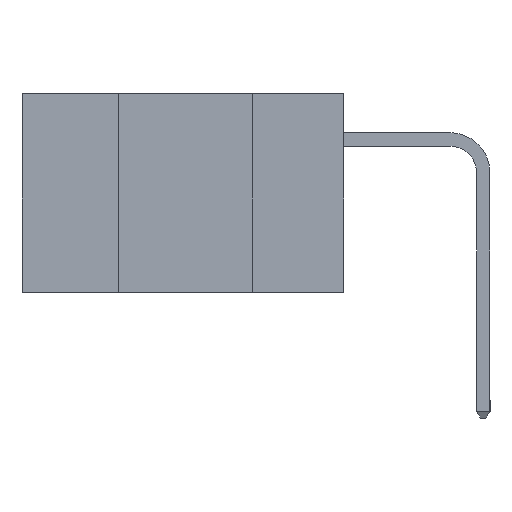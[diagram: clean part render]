
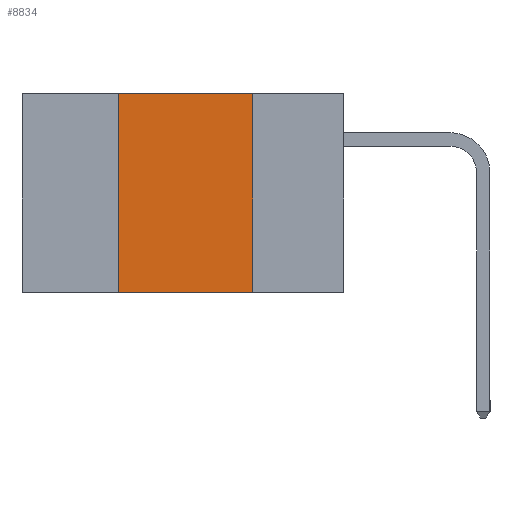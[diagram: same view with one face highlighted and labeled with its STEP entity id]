
A CAD part, left-side view. The second image highlights one B-rep face of the part: STEP entity #8834.
In plain terms, the highlighted planar face has unit normal (-1, 0, 0).
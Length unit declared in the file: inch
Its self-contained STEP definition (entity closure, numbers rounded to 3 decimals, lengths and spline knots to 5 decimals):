
#902 = DIRECTION ( 'NONE',  ( 0., 0., 1. ) ) ;
#1049 = VERTEX_POINT ( 'NONE', #13459 ) ;
#1389 = VECTOR ( 'NONE', #14288, 39.37008 ) ;
#2079 = CARTESIAN_POINT ( 'NONE',  ( 0., 0.42, -0.37 ) ) ;
#2468 = DIRECTION ( 'NONE',  ( 0., -1., 0. ) ) ;
#2486 = LINE ( 'NONE', #14290, #10947 ) ;
#2557 = CARTESIAN_POINT ( 'NONE',  ( 0., 0.17, -0.37 ) ) ;
#2605 = DIRECTION ( 'NONE',  ( 0., 0., -1. ) ) ;
#3822 = ORIENTED_EDGE ( 'NONE', *, *, #6301, .F. ) ;
#4528 = LINE ( 'NONE', #2079, #10556 ) ;
#4653 = ORIENTED_EDGE ( 'NONE', *, *, #6824, .T. ) ;
#5407 = VERTEX_POINT ( 'NONE', #14239 ) ;
#5997 = CARTESIAN_POINT ( 'NONE',  ( 0., 0.6, -0.37 ) ) ;
#6136 = AXIS2_PLACEMENT_3D ( 'NONE', #12160, #14434, #7365 ) ;
#6301 = EDGE_CURVE ( 'NONE', #1049, #13690, #12116, .T. ) ;
#6824 = EDGE_CURVE ( 'NONE', #5407, #13690, #13311, .T. ) ;
#6946 = FACE_OUTER_BOUND ( 'NONE', #10215, .T. ) ;
#7365 = DIRECTION ( 'NONE',  ( 0., 0., -1. ) ) ;
#8161 = VECTOR ( 'NONE', #2605, 39.37008 ) ;
#8766 = EDGE_CURVE ( 'NONE', #14682, #1049, #2486, .T. ) ;
#8834 = ADVANCED_FACE ( 'NONE', ( #6946 ), #13277, .F. ) ;
#10131 = CARTESIAN_POINT ( 'NONE',  ( 0., 0.42, 0. ) ) ;
#10215 = EDGE_LOOP ( 'NONE', ( #3822, #12230, #13303, #4653 ) ) ;
#10556 = VECTOR ( 'NONE', #902, 39.37008 ) ;
#10947 = VECTOR ( 'NONE', #2468, 39.37008 ) ;
#12116 = LINE ( 'NONE', #2557, #8161 ) ;
#12160 = CARTESIAN_POINT ( 'NONE',  ( 0., 0.6, 0. ) ) ;
#12230 = ORIENTED_EDGE ( 'NONE', *, *, #8766, .F. ) ;
#13277 = PLANE ( 'NONE',  #6136 ) ;
#13303 = ORIENTED_EDGE ( 'NONE', *, *, #14253, .F. ) ;
#13311 = LINE ( 'NONE', #5997, #1389 ) ;
#13459 = CARTESIAN_POINT ( 'NONE',  ( 0., 0.17, 0. ) ) ;
#13690 = VERTEX_POINT ( 'NONE', #14967 ) ;
#14239 = CARTESIAN_POINT ( 'NONE',  ( 0., 0.42, -0.37 ) ) ;
#14253 = EDGE_CURVE ( 'NONE', #5407, #14682, #4528, .T. ) ;
#14288 = DIRECTION ( 'NONE',  ( 0., -1., 0. ) ) ;
#14290 = CARTESIAN_POINT ( 'NONE',  ( 0., 0.6, 0. ) ) ;
#14434 = DIRECTION ( 'NONE',  ( 1., 0., 0. ) ) ;
#14682 = VERTEX_POINT ( 'NONE', #10131 ) ;
#14967 = CARTESIAN_POINT ( 'NONE',  ( 0., 0.17, -0.37 ) ) ;
